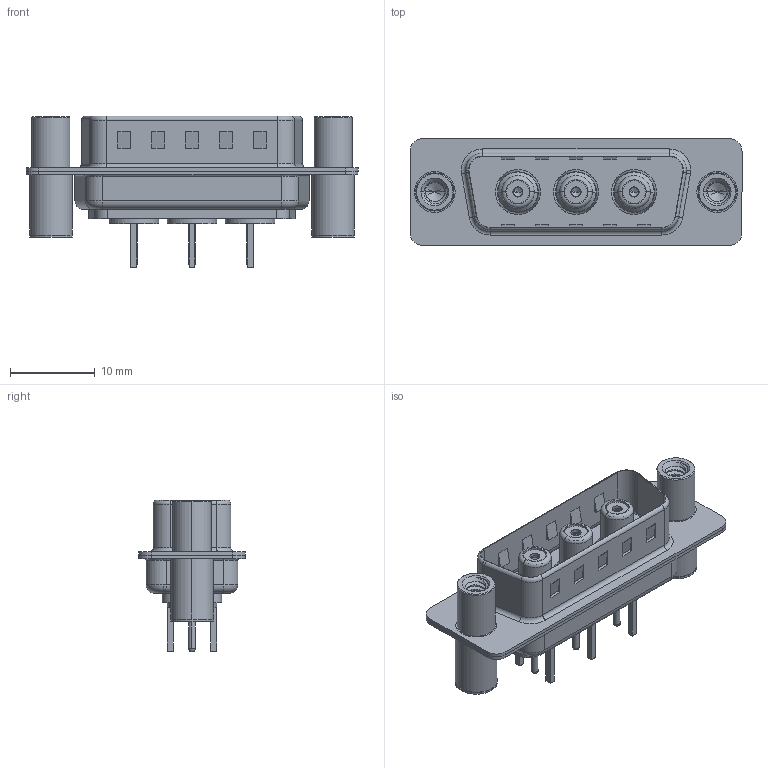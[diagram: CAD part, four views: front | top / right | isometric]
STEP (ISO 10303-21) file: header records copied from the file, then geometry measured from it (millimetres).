
FILE_DESCRIPTION (( 'STEP AP203' ), '1' );
FILE_NAME ('627-3W3-624-5T4.STEP', '2019-05-24T18:49:37', ( '' ), ( '' ), 'SwSTEP 2.0', 'SolidWorks 2016', '' );
FILE_SCHEMA (( 'CONFIG_CONTROL_DESIGN' ));
Length unit declared in the file: millimetre
Products named in the file (11): 627Combo Shell Front_15 Contacts; 627Combo Threaded Standoff and Board Spacer_4; Co-Ax Jack_Straight PC Tail; Socket_Str; Insulator Socket; Co-Ax Jack Assy_S; Insulator Socket 2; 627-3W3-624-5T4; Locking Collar; 627Combo Housing_3W3; 627Combo Shell Rear_15 Contacts
Assembly tree (13 placements, depth 3):
  627-3W3-624-5T4
    627Combo Housing_3W3
    627Combo Shell Rear_15 Contacts
    627Combo Shell Front_15 Contacts
    627Combo Threaded Standoff and Board Spacer_4  x2
    Co-Ax Jack Assy_S  x3
      Co-Ax Jack_Straight PC Tail
      Insulator Socket
      Insulator Socket 2
      Locking Collar
      Socket_Str
Bounding box: 39.15 x 12.6 x 17.9 mm (x, y, z)
Volume: 2194.5 mm3; surface area: 6449.6 mm2
Topology: 20 solids, 20 shells, 759 faces, 1830 edges, 1144 vertices
Faces by surface type: cylinder 326, plane 286, torus 66, cone 57, bspline 18, sphere 6
Entity records: 17258 total; most frequent: CARTESIAN_POINT 4766, DIRECTION 2435, ORIENTED_EDGE 2304, EDGE_CURVE 1152, AXIS2_PLACEMENT_3D 915, VERTEX_POINT 727, VECTOR 605, LINE 605
